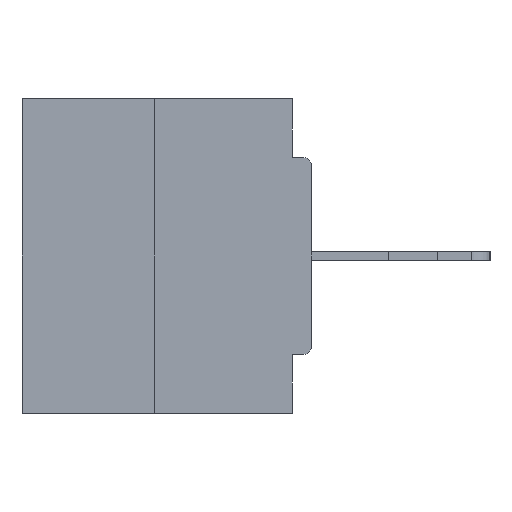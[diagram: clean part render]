
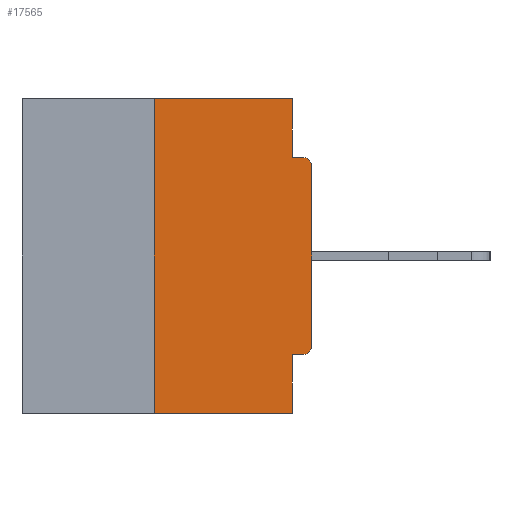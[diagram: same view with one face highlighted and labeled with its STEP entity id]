
A CAD part, left-side view. The second image highlights one B-rep face of the part: STEP entity #17565.
In plain terms, the highlighted planar face has unit normal (-1, 0, 0).
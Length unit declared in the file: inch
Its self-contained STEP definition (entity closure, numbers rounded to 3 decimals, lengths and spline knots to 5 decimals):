
#227 = VERTEX_POINT ( 'NONE', #33728 ) ;
#2137 = AXIS2_PLACEMENT_3D ( 'NONE', #27386, #13912, #36446 ) ;
#2195 = VERTEX_POINT ( 'NONE', #10035 ) ;
#3067 = DIRECTION ( 'NONE',  ( 0., -1., 0. ) ) ;
#3071 = ORIENTED_EDGE ( 'NONE', *, *, #3295, .F. ) ;
#3090 = ORIENTED_EDGE ( 'NONE', *, *, #35611, .F. ) ;
#3295 = EDGE_CURVE ( 'NONE', #2195, #4085, #20426, .T. ) ;
#3435 = LINE ( 'NONE', #22663, #5452 ) ;
#3812 = VERTEX_POINT ( 'NONE', #17982 ) ;
#4085 = VERTEX_POINT ( 'NONE', #25896 ) ;
#4278 = EDGE_CURVE ( 'NONE', #10451, #15016, #26979, .T. ) ;
#4326 = CARTESIAN_POINT ( 'NONE',  ( 0., 0.031, -0.0935 ) ) ;
#4628 = LINE ( 'NONE', #21440, #23436 ) ;
#4694 = EDGE_CURVE ( 'NONE', #10451, #4085, #32462, .T. ) ;
#4717 = DIRECTION ( 'NONE',  ( -1., 0., 0. ) ) ;
#5452 = VECTOR ( 'NONE', #3067, 39.37008 ) ;
#5502 = DIRECTION ( 'NONE',  ( 0., 0., -1. ) ) ;
#6483 = EDGE_CURVE ( 'NONE', #7806, #18187, #24301, .T. ) ;
#6487 = EDGE_LOOP ( 'NONE', ( #3090, #31258, #23761, #3071, #13658, #12784, #7543, #16466, #8328, #24639 ) ) ;
#6718 = AXIS2_PLACEMENT_3D ( 'NONE', #30006, #4717, #15994 ) ;
#6840 = DIRECTION ( 'NONE',  ( 0., 0., 1. ) ) ;
#7543 = ORIENTED_EDGE ( 'NONE', *, *, #7860, .T. ) ;
#7806 = VERTEX_POINT ( 'NONE', #17778 ) ;
#7860 = EDGE_CURVE ( 'NONE', #3812, #227, #31612, .T. ) ;
#8328 = ORIENTED_EDGE ( 'NONE', *, *, #23307, .F. ) ;
#9569 = DIRECTION ( 'NONE',  ( 0., -1., 0. ) ) ;
#10035 = CARTESIAN_POINT ( 'NONE',  ( 0., 0.031, -0.4065 ) ) ;
#10451 = VERTEX_POINT ( 'NONE', #29389 ) ;
#12329 = EDGE_CURVE ( 'NONE', #25335, #3812, #17510, .T. ) ;
#12635 = CIRCLE ( 'NONE', #6718, 0.015 ) ;
#12784 = ORIENTED_EDGE ( 'NONE', *, *, #12329, .T. ) ;
#12979 = LINE ( 'NONE', #35690, #24159 ) ;
#13273 = PLANE ( 'NONE',  #15295 ) ;
#13658 = ORIENTED_EDGE ( 'NONE', *, *, #15750, .F. ) ;
#13912 = DIRECTION ( 'NONE',  ( -1., 0., 0. ) ) ;
#15016 = VERTEX_POINT ( 'NONE', #27841 ) ;
#15295 = AXIS2_PLACEMENT_3D ( 'NONE', #25095, #19540, #5502 ) ;
#15397 = VECTOR ( 'NONE', #6840, 39.37008 ) ;
#15750 = EDGE_CURVE ( 'NONE', #25335, #2195, #4628, .T. ) ;
#15994 = DIRECTION ( 'NONE',  ( 0., 0., -1. ) ) ;
#16466 = ORIENTED_EDGE ( 'NONE', *, *, #30108, .T. ) ;
#16800 = VECTOR ( 'NONE', #22957, 39.37008 ) ;
#17510 = CIRCLE ( 'NONE', #2137, 0.015 ) ;
#17565 = ADVANCED_FACE ( 'NONE', ( #27665 ), #13273, .F. ) ;
#17778 = CARTESIAN_POINT ( 'NONE',  ( 0., 0.031, 0. ) ) ;
#17982 = CARTESIAN_POINT ( 'NONE',  ( 0., 0., -0.3915 ) ) ;
#18187 = VERTEX_POINT ( 'NONE', #4326 ) ;
#19540 = DIRECTION ( 'NONE',  ( 1., 0., 0. ) ) ;
#19825 = CARTESIAN_POINT ( 'NONE',  ( 0., 0., 0. ) ) ;
#20426 = LINE ( 'NONE', #31314, #34891 ) ;
#21440 = CARTESIAN_POINT ( 'NONE',  ( 0., 0., -0.4065 ) ) ;
#22663 = CARTESIAN_POINT ( 'NONE',  ( 0., 0., -0.0935 ) ) ;
#22957 = DIRECTION ( 'NONE',  ( 0., 0., 1. ) ) ;
#23307 = EDGE_CURVE ( 'NONE', #18187, #35545, #3435, .T. ) ;
#23436 = VECTOR ( 'NONE', #32694, 39.37008 ) ;
#23561 = DIRECTION ( 'NONE',  ( 0., 0., -1. ) ) ;
#23612 = CARTESIAN_POINT ( 'NONE',  ( 0., 0.46, -0.5 ) ) ;
#23761 = ORIENTED_EDGE ( 'NONE', *, *, #4694, .T. ) ;
#24159 = VECTOR ( 'NONE', #33074, 39.37008 ) ;
#24203 = CARTESIAN_POINT ( 'NONE',  ( 0., 0.25, 0. ) ) ;
#24301 = LINE ( 'NONE', #24482, #26743 ) ;
#24482 = CARTESIAN_POINT ( 'NONE',  ( 0., 0.031, 0. ) ) ;
#24639 = ORIENTED_EDGE ( 'NONE', *, *, #6483, .F. ) ;
#25095 = CARTESIAN_POINT ( 'NONE',  ( 0., 0.46, 0. ) ) ;
#25335 = VERTEX_POINT ( 'NONE', #31242 ) ;
#25896 = CARTESIAN_POINT ( 'NONE',  ( 0., 0.031, -0.5 ) ) ;
#26743 = VECTOR ( 'NONE', #33331, 39.37008 ) ;
#26979 = LINE ( 'NONE', #24203, #15397 ) ;
#27386 = CARTESIAN_POINT ( 'NONE',  ( 0., 0.015, -0.3915 ) ) ;
#27665 = FACE_OUTER_BOUND ( 'NONE', #6487, .T. ) ;
#27841 = CARTESIAN_POINT ( 'NONE',  ( 0., 0.25, 0. ) ) ;
#29389 = CARTESIAN_POINT ( 'NONE',  ( 0., 0.25, -0.5 ) ) ;
#30006 = CARTESIAN_POINT ( 'NONE',  ( 0., 0.015, -0.1085 ) ) ;
#30108 = EDGE_CURVE ( 'NONE', #227, #35545, #12635, .T. ) ;
#31242 = CARTESIAN_POINT ( 'NONE',  ( 0., 0.015, -0.4065 ) ) ;
#31258 = ORIENTED_EDGE ( 'NONE', *, *, #4278, .F. ) ;
#31314 = CARTESIAN_POINT ( 'NONE',  ( 0., 0.031, -0.5 ) ) ;
#31331 = VECTOR ( 'NONE', #9569, 39.37008 ) ;
#31612 = LINE ( 'NONE', #19825, #16800 ) ;
#32462 = LINE ( 'NONE', #23612, #31331 ) ;
#32694 = DIRECTION ( 'NONE',  ( 0., 1., 0. ) ) ;
#33074 = DIRECTION ( 'NONE',  ( 0., -1., 0. ) ) ;
#33331 = DIRECTION ( 'NONE',  ( 0., 0., -1. ) ) ;
#33728 = CARTESIAN_POINT ( 'NONE',  ( 0., 0., -0.1085 ) ) ;
#34891 = VECTOR ( 'NONE', #23561, 39.37008 ) ;
#35545 = VERTEX_POINT ( 'NONE', #35861 ) ;
#35611 = EDGE_CURVE ( 'NONE', #15016, #7806, #12979, .T. ) ;
#35690 = CARTESIAN_POINT ( 'NONE',  ( 0., 0.46, 0. ) ) ;
#35861 = CARTESIAN_POINT ( 'NONE',  ( 0., 0.015, -0.0935 ) ) ;
#36446 = DIRECTION ( 'NONE',  ( 0., 0., -1. ) ) ;
